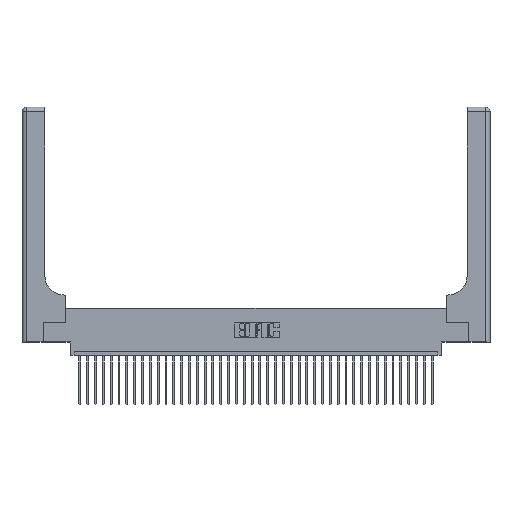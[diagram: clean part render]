
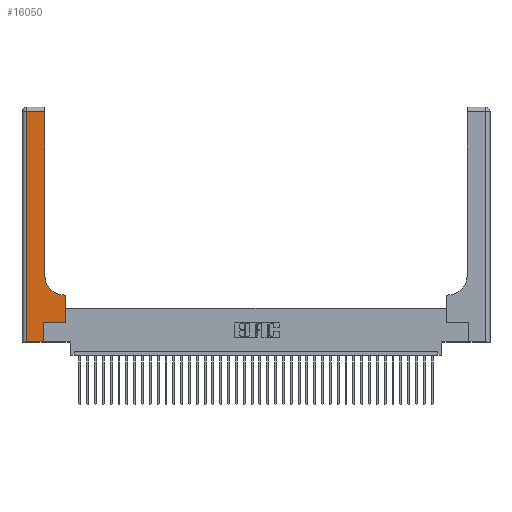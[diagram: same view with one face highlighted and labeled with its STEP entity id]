
A CAD part, top view. The second image highlights one B-rep face of the part: STEP entity #16050.
In plain terms, the highlighted planar face has unit normal (0, 0, 1).
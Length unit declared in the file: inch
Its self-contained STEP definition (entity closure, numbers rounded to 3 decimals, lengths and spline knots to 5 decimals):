
#45 = LINE ( 'NONE', #24565, #31474 ) ;
#62 = VECTOR ( 'NONE', #32431, 39.37008 ) ;
#219 = LINE ( 'NONE', #33532, #28393 ) ;
#474 = ORIENTED_EDGE ( 'NONE', *, *, #16128, .T. ) ;
#599 = LINE ( 'NONE', #37708, #18751 ) ;
#2049 = DIRECTION ( 'NONE',  ( 1., 0., 0. ) ) ;
#2513 = VECTOR ( 'NONE', #22494, 39.37008 ) ;
#2650 = CARTESIAN_POINT ( 'NONE',  ( 0.2915, 2.94, 0.37 ) ) ;
#3037 = VERTEX_POINT ( 'NONE', #5518 ) ;
#4226 = EDGE_CURVE ( 'NONE', #6372, #31059, #219, .T. ) ;
#4684 = DIRECTION ( 'NONE',  ( 0., -1., 0. ) ) ;
#5328 = LINE ( 'NONE', #29259, #62 ) ;
#5451 = VECTOR ( 'NONE', #4684, 39.37008 ) ;
#5505 = ORIENTED_EDGE ( 'NONE', *, *, #20593, .T. ) ;
#5518 = CARTESIAN_POINT ( 'NONE',  ( 0.269, 0.25, 0.37 ) ) ;
#6005 = AXIS2_PLACEMENT_3D ( 'NONE', #21431, #6486, #31103 ) ;
#6372 = VERTEX_POINT ( 'NONE', #34457 ) ;
#6486 = DIRECTION ( 'NONE',  ( 0., 0., -1. ) ) ;
#7498 = EDGE_LOOP ( 'NONE', ( #37489, #30244, #37907, #8332, #8019, #15862, #5505, #474, #33056 ) ) ;
#8019 = ORIENTED_EDGE ( 'NONE', *, *, #8760, .T. ) ;
#8332 = ORIENTED_EDGE ( 'NONE', *, *, #4226, .T. ) ;
#8354 = EDGE_CURVE ( 'NONE', #24940, #6372, #35462, .T. ) ;
#8569 = CARTESIAN_POINT ( 'NONE',  ( 0.5415, 0.6, 0.37 ) ) ;
#8760 = EDGE_CURVE ( 'NONE', #31059, #3037, #599, .T. ) ;
#9863 = LINE ( 'NONE', #19641, #11770 ) ;
#10062 = FACE_OUTER_BOUND ( 'NONE', #7498, .T. ) ;
#11527 = VERTEX_POINT ( 'NONE', #17222 ) ;
#11770 = VECTOR ( 'NONE', #2049, 39.37008 ) ;
#12028 = EDGE_CURVE ( 'NONE', #3037, #28581, #9863, .T. ) ;
#12995 = CIRCLE ( 'NONE', #6005, 0.25 ) ;
#13992 = CARTESIAN_POINT ( 'NONE',  ( 0.06, 2.94, 0.37 ) ) ;
#14643 = PLANE ( 'NONE',  #18545 ) ;
#14879 = VERTEX_POINT ( 'NONE', #8569 ) ;
#15471 = EDGE_CURVE ( 'NONE', #25103, #24940, #27754, .T. ) ;
#15862 = ORIENTED_EDGE ( 'NONE', *, *, #12028, .T. ) ;
#16050 = ADVANCED_FACE ( 'NONE', ( #10062 ), #14643, .F. ) ;
#16128 = EDGE_CURVE ( 'NONE', #11527, #14879, #45, .T. ) ;
#16445 = VERTEX_POINT ( 'NONE', #22760 ) ;
#17222 = CARTESIAN_POINT ( 'NONE',  ( 0.5585, 0.6, 0.37 ) ) ;
#18545 = AXIS2_PLACEMENT_3D ( 'NONE', #32723, #35903, #29407 ) ;
#18751 = VECTOR ( 'NONE', #19287, 39.37008 ) ;
#19263 = CARTESIAN_POINT ( 'NONE',  ( 0.5585, 0.25, 0.37 ) ) ;
#19287 = DIRECTION ( 'NONE',  ( 0., 1., 0. ) ) ;
#19641 = CARTESIAN_POINT ( 'NONE',  ( 0.269, 0.25, 0.37 ) ) ;
#20593 = EDGE_CURVE ( 'NONE', #28581, #11527, #5328, .T. ) ;
#21236 = VECTOR ( 'NONE', #31208, 39.37008 ) ;
#21431 = CARTESIAN_POINT ( 'NONE',  ( 0.5415, 0.85, 0.37 ) ) ;
#22368 = CARTESIAN_POINT ( 'NONE',  ( 0., 2.94, 0.37 ) ) ;
#22494 = DIRECTION ( 'NONE',  ( -1., 0., 0. ) ) ;
#22760 = CARTESIAN_POINT ( 'NONE',  ( 0.2915, 0.85, 0.37 ) ) ;
#22927 = CARTESIAN_POINT ( 'NONE',  ( 0.06, 3., 0.37 ) ) ;
#24565 = CARTESIAN_POINT ( 'NONE',  ( 0.2915, 0.6, 0.37 ) ) ;
#24940 = VERTEX_POINT ( 'NONE', #13992 ) ;
#25103 = VERTEX_POINT ( 'NONE', #2650 ) ;
#25315 = EDGE_CURVE ( 'NONE', #16445, #25103, #28861, .T. ) ;
#27754 = LINE ( 'NONE', #22368, #2513 ) ;
#28393 = VECTOR ( 'NONE', #30336, 39.37008 ) ;
#28581 = VERTEX_POINT ( 'NONE', #19263 ) ;
#28717 = CARTESIAN_POINT ( 'NONE',  ( 0.2915, 3., 0.37 ) ) ;
#28861 = LINE ( 'NONE', #28717, #21236 ) ;
#29259 = CARTESIAN_POINT ( 'NONE',  ( 0.5585, 0.25, 0.37 ) ) ;
#29407 = DIRECTION ( 'NONE',  ( -1., 0., 0. ) ) ;
#30244 = ORIENTED_EDGE ( 'NONE', *, *, #15471, .T. ) ;
#30336 = DIRECTION ( 'NONE',  ( 1., 0., 0. ) ) ;
#31059 = VERTEX_POINT ( 'NONE', #35514 ) ;
#31103 = DIRECTION ( 'NONE',  ( 1., 0., 0. ) ) ;
#31208 = DIRECTION ( 'NONE',  ( 0., 1., 0. ) ) ;
#31474 = VECTOR ( 'NONE', #36884, 39.37008 ) ;
#32431 = DIRECTION ( 'NONE',  ( 0., 1., 0. ) ) ;
#32723 = CARTESIAN_POINT ( 'NONE',  ( 0., 3., 0.37 ) ) ;
#33056 = ORIENTED_EDGE ( 'NONE', *, *, #37791, .T. ) ;
#33532 = CARTESIAN_POINT ( 'NONE',  ( 0., 0., 0.37 ) ) ;
#34457 = CARTESIAN_POINT ( 'NONE',  ( 0.06, 0., 0.37 ) ) ;
#35462 = LINE ( 'NONE', #22927, #5451 ) ;
#35514 = CARTESIAN_POINT ( 'NONE',  ( 0.269, 0., 0.37 ) ) ;
#35903 = DIRECTION ( 'NONE',  ( 0., 0., -1. ) ) ;
#36884 = DIRECTION ( 'NONE',  ( -1., 0., 0. ) ) ;
#37489 = ORIENTED_EDGE ( 'NONE', *, *, #25315, .T. ) ;
#37708 = CARTESIAN_POINT ( 'NONE',  ( 0.269, 0., 0.37 ) ) ;
#37791 = EDGE_CURVE ( 'NONE', #14879, #16445, #12995, .T. ) ;
#37907 = ORIENTED_EDGE ( 'NONE', *, *, #8354, .T. ) ;
